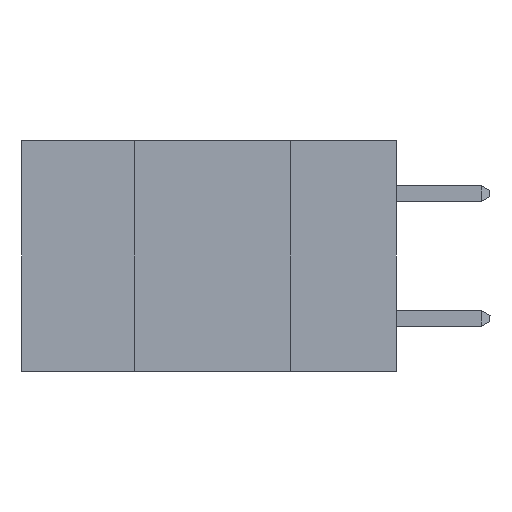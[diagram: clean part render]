
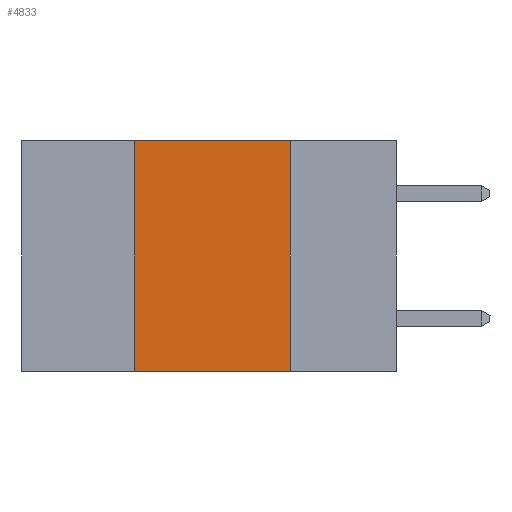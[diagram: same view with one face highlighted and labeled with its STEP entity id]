
A CAD part, left-side view. The second image highlights one B-rep face of the part: STEP entity #4833.
In plain terms, the highlighted planar face has unit normal (-1, 0, 0).
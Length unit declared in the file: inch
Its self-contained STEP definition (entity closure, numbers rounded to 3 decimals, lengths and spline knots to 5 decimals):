
#52 = DIRECTION ( 'NONE',  ( 0., 0., -1. ) ) ;
#174 = VECTOR ( 'NONE', #8366, 39.37008 ) ;
#641 = CARTESIAN_POINT ( 'NONE',  ( 0., 0.42, -0.37 ) ) ;
#2007 = VERTEX_POINT ( 'NONE', #641 ) ;
#2144 = FACE_OUTER_BOUND ( 'NONE', #33741, .T. ) ;
#2892 = DIRECTION ( 'NONE',  ( 0., -1., 0. ) ) ;
#3122 = ORIENTED_EDGE ( 'NONE', *, *, #14238, .T. ) ;
#3793 = LINE ( 'NONE', #23093, #5026 ) ;
#3849 = EDGE_CURVE ( 'NONE', #31410, #22404, #16207, .T. ) ;
#4833 = ADVANCED_FACE ( 'NONE', ( #2144 ), #21271, .F. ) ;
#5026 = VECTOR ( 'NONE', #2892, 39.37008 ) ;
#5392 = ORIENTED_EDGE ( 'NONE', *, *, #10814, .F. ) ;
#5682 = CARTESIAN_POINT ( 'NONE',  ( 0., 0.6, 0. ) ) ;
#8306 = DIRECTION ( 'NONE',  ( 1., 0., 0. ) ) ;
#8366 = DIRECTION ( 'NONE',  ( 0., 0., -1. ) ) ;
#8987 = ORIENTED_EDGE ( 'NONE', *, *, #3849, .F. ) ;
#10027 = ORIENTED_EDGE ( 'NONE', *, *, #27801, .F. ) ;
#10814 = EDGE_CURVE ( 'NONE', #32994, #31410, #3793, .T. ) ;
#13660 = CARTESIAN_POINT ( 'NONE',  ( 0., 0.17, 0. ) ) ;
#14238 = EDGE_CURVE ( 'NONE', #2007, #22404, #24664, .T. ) ;
#16207 = LINE ( 'NONE', #13660, #174 ) ;
#16431 = CARTESIAN_POINT ( 'NONE',  ( 0., 0.42, 0. ) ) ;
#21271 = PLANE ( 'NONE',  #22516 ) ;
#21485 = CARTESIAN_POINT ( 'NONE',  ( 0., 0.6, -0.37 ) ) ;
#21820 = DIRECTION ( 'NONE',  ( 0., -1., 0. ) ) ;
#22404 = VERTEX_POINT ( 'NONE', #27816 ) ;
#22516 = AXIS2_PLACEMENT_3D ( 'NONE', #5682, #8306, #52 ) ;
#22705 = LINE ( 'NONE', #26110, #30461 ) ;
#23093 = CARTESIAN_POINT ( 'NONE',  ( 0., 0.6, 0. ) ) ;
#23139 = CARTESIAN_POINT ( 'NONE',  ( 0., 0.17, 0. ) ) ;
#24664 = LINE ( 'NONE', #21485, #30810 ) ;
#26110 = CARTESIAN_POINT ( 'NONE',  ( 0., 0.42, 0. ) ) ;
#27801 = EDGE_CURVE ( 'NONE', #2007, #32994, #22705, .T. ) ;
#27816 = CARTESIAN_POINT ( 'NONE',  ( 0., 0.17, -0.37 ) ) ;
#28503 = DIRECTION ( 'NONE',  ( 0., 0., 1. ) ) ;
#30461 = VECTOR ( 'NONE', #28503, 39.37008 ) ;
#30810 = VECTOR ( 'NONE', #21820, 39.37008 ) ;
#31410 = VERTEX_POINT ( 'NONE', #23139 ) ;
#32994 = VERTEX_POINT ( 'NONE', #16431 ) ;
#33741 = EDGE_LOOP ( 'NONE', ( #8987, #5392, #10027, #3122 ) ) ;
